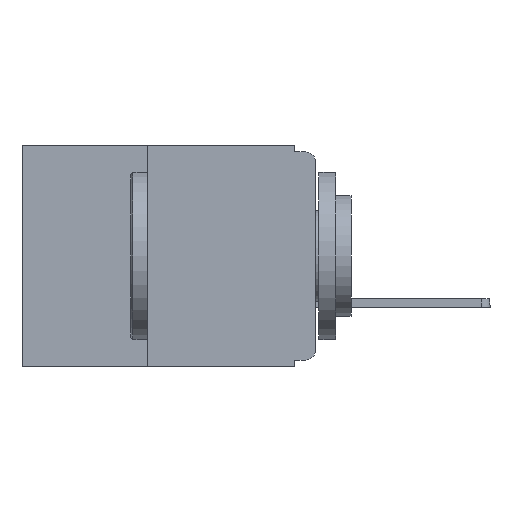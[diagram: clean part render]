
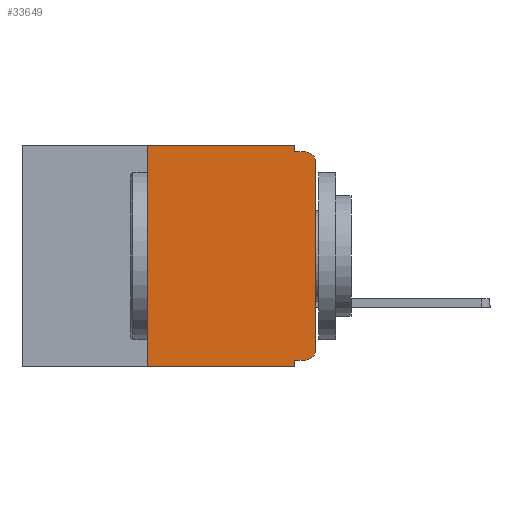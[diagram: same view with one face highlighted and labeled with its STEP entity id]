
A CAD part, left-side view. The second image highlights one B-rep face of the part: STEP entity #33649.
In plain terms, the highlighted planar face has unit normal (-1, 0, 0).
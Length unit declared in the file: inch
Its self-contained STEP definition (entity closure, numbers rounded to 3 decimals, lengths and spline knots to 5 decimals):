
#245 = LINE ( 'NONE', #33620, #27275 ) ;
#1240 = DIRECTION ( 'NONE',  ( 0., 1., 0. ) ) ;
#1298 = PLANE ( 'NONE',  #32338 ) ;
#1720 = EDGE_CURVE ( 'NONE', #13466, #9513, #19267, .T. ) ;
#1849 = VECTOR ( 'NONE', #23083, 39.37008 ) ;
#2211 = ORIENTED_EDGE ( 'NONE', *, *, #1720, .T. ) ;
#2820 = ORIENTED_EDGE ( 'NONE', *, *, #11056, .T. ) ;
#3243 = CIRCLE ( 'NONE', #22111, 0.015 ) ;
#3247 = DIRECTION ( 'NONE',  ( -1., 0., 0. ) ) ;
#3826 = CARTESIAN_POINT ( 'NONE',  ( 0., 0., -0.32 ) ) ;
#4100 = VERTEX_POINT ( 'NONE', #30796 ) ;
#4604 = EDGE_CURVE ( 'NONE', #9542, #9513, #18646, .T. ) ;
#4708 = CARTESIAN_POINT ( 'NONE',  ( 0., 0.437, 0. ) ) ;
#4904 = VECTOR ( 'NONE', #1240, 39.37008 ) ;
#5927 = VERTEX_POINT ( 'NONE', #13541 ) ;
#6239 = VERTEX_POINT ( 'NONE', #20607 ) ;
#6826 = ORIENTED_EDGE ( 'NONE', *, *, #24047, .T. ) ;
#7798 = CARTESIAN_POINT ( 'NONE',  ( 0., 0.25, -0.33 ) ) ;
#7842 = VECTOR ( 'NONE', #28807, 39.37008 ) ;
#8305 = AXIS2_PLACEMENT_3D ( 'NONE', #18909, #3247, #21602 ) ;
#9513 = VERTEX_POINT ( 'NONE', #31105 ) ;
#9542 = VERTEX_POINT ( 'NONE', #31210 ) ;
#9742 = VECTOR ( 'NONE', #17164, 39.37008 ) ;
#11056 = EDGE_CURVE ( 'NONE', #28217, #5927, #11373, .T. ) ;
#11373 = LINE ( 'NONE', #27631, #9742 ) ;
#12105 = CARTESIAN_POINT ( 'NONE',  ( 0., 0.437, -0.33 ) ) ;
#12677 = DIRECTION ( 'NONE',  ( -1., 0., 0. ) ) ;
#12745 = DIRECTION ( 'NONE',  ( 0., -1., 0. ) ) ;
#13143 = CARTESIAN_POINT ( 'NONE',  ( 0., 0.015, -0.32 ) ) ;
#13466 = VERTEX_POINT ( 'NONE', #28102 ) ;
#13501 = EDGE_CURVE ( 'NONE', #4100, #14546, #15729, .T. ) ;
#13541 = CARTESIAN_POINT ( 'NONE',  ( 0., 0., -0.025 ) ) ;
#14432 = CARTESIAN_POINT ( 'NONE',  ( 0., 0.437, 0. ) ) ;
#14546 = VERTEX_POINT ( 'NONE', #24140 ) ;
#14570 = CARTESIAN_POINT ( 'NONE',  ( 0., 0.031, -0.01 ) ) ;
#14698 = CIRCLE ( 'NONE', #8305, 0.015 ) ;
#15661 = EDGE_CURVE ( 'NONE', #13466, #4100, #26470, .T. ) ;
#15729 = LINE ( 'NONE', #4708, #1849 ) ;
#15770 = DIRECTION ( 'NONE',  ( 0., 0., 1. ) ) ;
#16631 = ORIENTED_EDGE ( 'NONE', *, *, #4604, .F. ) ;
#17054 = DIRECTION ( 'NONE',  ( 0., 0., -1. ) ) ;
#17164 = DIRECTION ( 'NONE',  ( 0., 0., 1. ) ) ;
#18332 = CARTESIAN_POINT ( 'NONE',  ( 0., 0., -0.01 ) ) ;
#18646 = LINE ( 'NONE', #18881, #24024 ) ;
#18823 = LINE ( 'NONE', #3826, #4904 ) ;
#18881 = CARTESIAN_POINT ( 'NONE',  ( 0., 0.031, -0.33 ) ) ;
#18909 = CARTESIAN_POINT ( 'NONE',  ( 0., 0.015, -0.305 ) ) ;
#19114 = ORIENTED_EDGE ( 'NONE', *, *, #27156, .F. ) ;
#19119 = DIRECTION ( 'NONE',  ( 0., 0., -1. ) ) ;
#19267 = LINE ( 'NONE', #12105, #25444 ) ;
#19659 = VERTEX_POINT ( 'NONE', #14570 ) ;
#20274 = VECTOR ( 'NONE', #15770, 39.37008 ) ;
#20607 = CARTESIAN_POINT ( 'NONE',  ( 0., 0.015, -0.01 ) ) ;
#20752 = FACE_OUTER_BOUND ( 'NONE', #24791, .T. ) ;
#21602 = DIRECTION ( 'NONE',  ( 0., 0., -1. ) ) ;
#22111 = AXIS2_PLACEMENT_3D ( 'NONE', #28380, #12677, #30958 ) ;
#23083 = DIRECTION ( 'NONE',  ( 0., -1., 0. ) ) ;
#23306 = EDGE_CURVE ( 'NONE', #5927, #6239, #3243, .T. ) ;
#23330 = DIRECTION ( 'NONE',  ( 0., 0., -1. ) ) ;
#23597 = ORIENTED_EDGE ( 'NONE', *, *, #29694, .F. ) ;
#24024 = VECTOR ( 'NONE', #19119, 39.37008 ) ;
#24047 = EDGE_CURVE ( 'NONE', #32680, #28217, #14698, .T. ) ;
#24140 = CARTESIAN_POINT ( 'NONE',  ( 0., 0.031, 0. ) ) ;
#24791 = EDGE_LOOP ( 'NONE', ( #2820, #28883, #30517, #23597, #29952, #32797, #2211, #16631, #19114, #6826 ) ) ;
#25444 = VECTOR ( 'NONE', #12745, 39.37008 ) ;
#25786 = EDGE_CURVE ( 'NONE', #19659, #6239, #28746, .T. ) ;
#26470 = LINE ( 'NONE', #7798, #20274 ) ;
#27156 = EDGE_CURVE ( 'NONE', #32680, #9542, #18823, .T. ) ;
#27275 = VECTOR ( 'NONE', #23330, 39.37008 ) ;
#27631 = CARTESIAN_POINT ( 'NONE',  ( 0., 0., 0. ) ) ;
#28102 = CARTESIAN_POINT ( 'NONE',  ( 0., 0.25, -0.33 ) ) ;
#28217 = VERTEX_POINT ( 'NONE', #32607 ) ;
#28380 = CARTESIAN_POINT ( 'NONE',  ( 0., 0.015, -0.025 ) ) ;
#28746 = LINE ( 'NONE', #18332, #7842 ) ;
#28807 = DIRECTION ( 'NONE',  ( 0., -1., 0. ) ) ;
#28883 = ORIENTED_EDGE ( 'NONE', *, *, #23306, .T. ) ;
#29694 = EDGE_CURVE ( 'NONE', #14546, #19659, #245, .T. ) ;
#29952 = ORIENTED_EDGE ( 'NONE', *, *, #13501, .F. ) ;
#30517 = ORIENTED_EDGE ( 'NONE', *, *, #25786, .F. ) ;
#30796 = CARTESIAN_POINT ( 'NONE',  ( 0., 0.25, 0. ) ) ;
#30958 = DIRECTION ( 'NONE',  ( 0., 0., -1. ) ) ;
#31105 = CARTESIAN_POINT ( 'NONE',  ( 0., 0.031, -0.33 ) ) ;
#31210 = CARTESIAN_POINT ( 'NONE',  ( 0., 0.031, -0.32 ) ) ;
#32338 = AXIS2_PLACEMENT_3D ( 'NONE', #14432, #32709, #17054 ) ;
#32607 = CARTESIAN_POINT ( 'NONE',  ( 0., 0., -0.305 ) ) ;
#32680 = VERTEX_POINT ( 'NONE', #13143 ) ;
#32709 = DIRECTION ( 'NONE',  ( 1., 0., 0. ) ) ;
#32797 = ORIENTED_EDGE ( 'NONE', *, *, #15661, .F. ) ;
#33620 = CARTESIAN_POINT ( 'NONE',  ( 0., 0.031, 0. ) ) ;
#33649 = ADVANCED_FACE ( 'NONE', ( #20752 ), #1298, .F. ) ;
